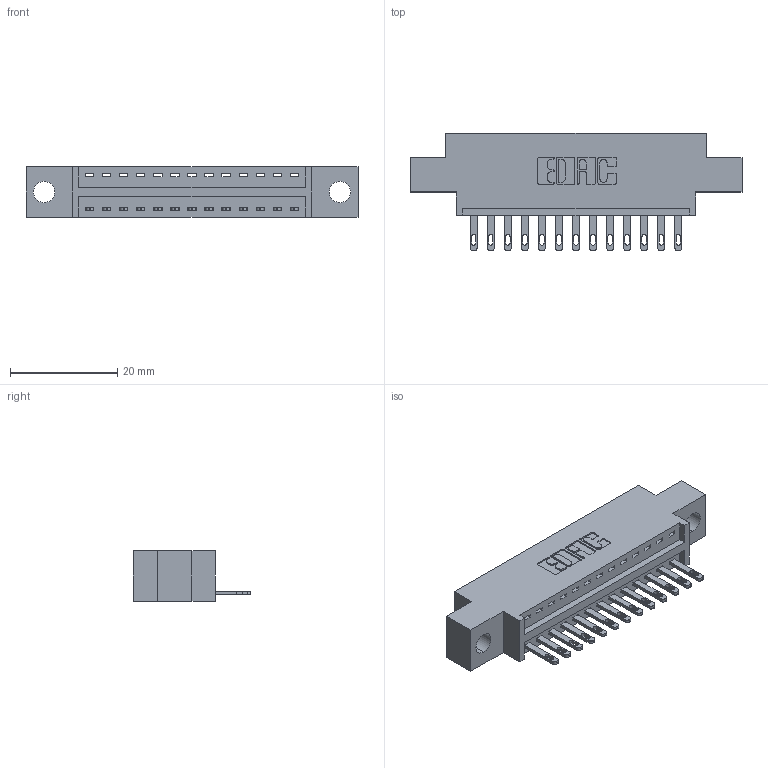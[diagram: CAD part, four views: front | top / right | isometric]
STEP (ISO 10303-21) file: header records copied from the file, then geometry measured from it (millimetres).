
FILE_DESCRIPTION (( 'STEP AP203' ), '1' );
FILE_NAME ('346-013-500-604.STEP', '2018-08-19T23:27:14', ( '' ), ( '' ), 'SwSTEP 2.0', 'SolidWorks 2016', '' );
FILE_SCHEMA (( 'CONFIG_CONTROL_DESIGN' ));
Length unit declared in the file: inch
Products named in the file (3): 346 Part_0.170 Offset - 0.156 Dia-TH; 345-292-001_345-293-100; 346-013-500-604
Assembly tree (14 placements, depth 2):
  346-013-500-604
    346 Part_0.170 Offset - 0.156 Dia-TH
    345-292-001_345-293-100  x13
Bounding box: 61.85 x 21.84 x 9.4 mm (x, y, z)
Volume: 5486.1 mm3; surface area: 6539.6 mm2
Topology: 14 solids, 14 shells, 828 faces, 2525 edges, 1682 vertices
Faces by surface type: plane 522, cylinder 306
Entity records: 12037 total; most frequent: CARTESIAN_POINT 2079, ORIENTED_EDGE 2026, DIRECTION 1871, EDGE_CURVE 1013, LINE 825, VECTOR 825, VERTEX_POINT 674, AXIS2_PLACEMENT_3D 523
